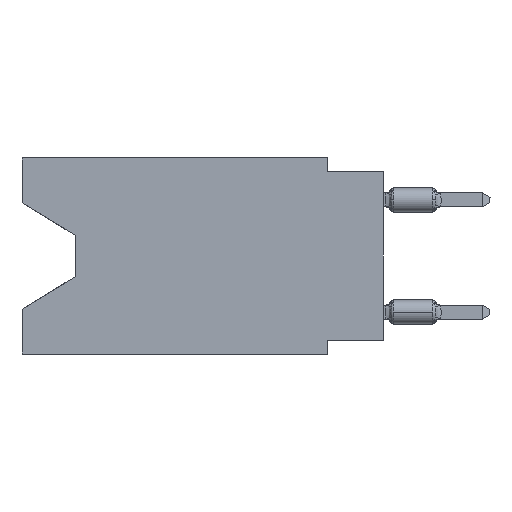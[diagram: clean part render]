
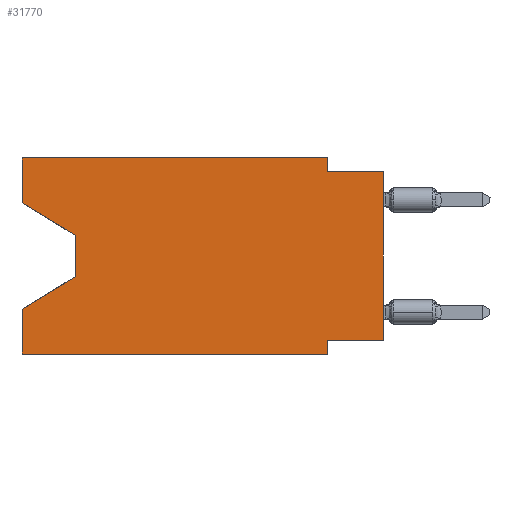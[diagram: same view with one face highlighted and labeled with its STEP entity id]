
A CAD part, left-side view. The second image highlights one B-rep face of the part: STEP entity #31770.
In plain terms, the highlighted planar face has unit normal (-1, 0, 0).
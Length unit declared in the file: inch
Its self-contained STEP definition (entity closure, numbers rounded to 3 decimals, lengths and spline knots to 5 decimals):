
#386 = DIRECTION ( 'NONE',  ( 1., 0., 0. ) ) ;
#463 = DIRECTION ( 'NONE',  ( 0., 0., 1. ) ) ;
#1813 = VECTOR ( 'NONE', #39213, 39.37008 ) ;
#2284 = VERTEX_POINT ( 'NONE', #43591 ) ;
#3440 = EDGE_CURVE ( 'NONE', #39043, #18679, #49309, .T. ) ;
#3689 = ORIENTED_EDGE ( 'NONE', *, *, #38426, .F. ) ;
#4699 = VECTOR ( 'NONE', #14234, 39.37008 ) ;
#5346 = CARTESIAN_POINT ( 'NONE',  ( 0., 0.645, -0.08025 ) ) ;
#5384 = CARTESIAN_POINT ( 'NONE',  ( 0., 0.1, -0.025 ) ) ;
#5559 = ORIENTED_EDGE ( 'NONE', *, *, #10562, .T. ) ;
#5564 = CARTESIAN_POINT ( 'NONE',  ( 0., 0.1, -0.35 ) ) ;
#5602 = DIRECTION ( 'NONE',  ( 0., -1., 0. ) ) ;
#5837 = LINE ( 'NONE', #22225, #13794 ) ;
#6562 = CARTESIAN_POINT ( 'NONE',  ( 0., 0.1, -0.35 ) ) ;
#6981 = CARTESIAN_POINT ( 'NONE',  ( 0., 0.645, -0.35 ) ) ;
#7416 = LINE ( 'NONE', #23812, #23748 ) ;
#8357 = EDGE_CURVE ( 'NONE', #27880, #24986, #37731, .T. ) ;
#8923 = DIRECTION ( 'NONE',  ( 0., 0., 1. ) ) ;
#9440 = LINE ( 'NONE', #12428, #40770 ) ;
#9547 = VECTOR ( 'NONE', #10209, 39.37008 ) ;
#9604 = LINE ( 'NONE', #26022, #52636 ) ;
#9800 = VERTEX_POINT ( 'NONE', #5564 ) ;
#10209 = DIRECTION ( 'NONE',  ( 0., 0., 1. ) ) ;
#10562 = EDGE_CURVE ( 'NONE', #45503, #2284, #9440, .T. ) ;
#10988 = VERTEX_POINT ( 'NONE', #50280 ) ;
#12251 = VECTOR ( 'NONE', #8923, 39.37008 ) ;
#12428 = CARTESIAN_POINT ( 'NONE',  ( 0., 0.55, -0.212 ) ) ;
#13794 = VECTOR ( 'NONE', #26280, 39.37008 ) ;
#13832 = ORIENTED_EDGE ( 'NONE', *, *, #48872, .F. ) ;
#14234 = DIRECTION ( 'NONE',  ( 0., -1., 0. ) ) ;
#15214 = LINE ( 'NONE', #22788, #1813 ) ;
#16140 = VERTEX_POINT ( 'NONE', #45741 ) ;
#16524 = DIRECTION ( 'NONE',  ( 0., 1., 0. ) ) ;
#18679 = VERTEX_POINT ( 'NONE', #5384 ) ;
#18775 = LINE ( 'NONE', #43043, #4699 ) ;
#19241 = VECTOR ( 'NONE', #21773, 39.37008 ) ;
#20510 = CARTESIAN_POINT ( 'NONE',  ( 0., 0.645, 0. ) ) ;
#21499 = CARTESIAN_POINT ( 'NONE',  ( 0., 0.55, -0.138 ) ) ;
#21773 = DIRECTION ( 'NONE',  ( 0., 0., -1. ) ) ;
#22225 = CARTESIAN_POINT ( 'NONE',  ( 0., 0.645, -0.35 ) ) ;
#22643 = ORIENTED_EDGE ( 'NONE', *, *, #25276, .T. ) ;
#22788 = CARTESIAN_POINT ( 'NONE',  ( 0., 0.645, -0.08025 ) ) ;
#23230 = ORIENTED_EDGE ( 'NONE', *, *, #36352, .F. ) ;
#23360 = ORIENTED_EDGE ( 'NONE', *, *, #43821, .T. ) ;
#23748 = VECTOR ( 'NONE', #16524, 39.37008 ) ;
#23812 = CARTESIAN_POINT ( 'NONE',  ( 0., 0., -0.325 ) ) ;
#24648 = ORIENTED_EDGE ( 'NONE', *, *, #8357, .T. ) ;
#24986 = VERTEX_POINT ( 'NONE', #38938 ) ;
#25276 = EDGE_CURVE ( 'NONE', #16140, #45503, #30129, .T. ) ;
#26022 = CARTESIAN_POINT ( 'NONE',  ( 0., 0.645, 0. ) ) ;
#26280 = DIRECTION ( 'NONE',  ( 0., -1., 0. ) ) ;
#26808 = CARTESIAN_POINT ( 'NONE',  ( 0., 0.1, 0. ) ) ;
#26828 = ORIENTED_EDGE ( 'NONE', *, *, #41934, .T. ) ;
#27648 = VECTOR ( 'NONE', #43235, 39.37008 ) ;
#27691 = VERTEX_POINT ( 'NONE', #6981 ) ;
#27880 = VERTEX_POINT ( 'NONE', #36312 ) ;
#28951 = LINE ( 'NONE', #49660, #36181 ) ;
#30027 = ORIENTED_EDGE ( 'NONE', *, *, #42074, .F. ) ;
#30129 = LINE ( 'NONE', #21499, #19241 ) ;
#31222 = ORIENTED_EDGE ( 'NONE', *, *, #41468, .F. ) ;
#31770 = ADVANCED_FACE ( 'NONE', ( #40521 ), #52617, .F. ) ;
#32795 = VERTEX_POINT ( 'NONE', #5346 ) ;
#33426 = CARTESIAN_POINT ( 'NONE',  ( 0., 0., 0. ) ) ;
#33681 = DIRECTION ( 'NONE',  ( 0., 0.855, -0.519 ) ) ;
#36181 = VECTOR ( 'NONE', #463, 39.37008 ) ;
#36312 = CARTESIAN_POINT ( 'NONE',  ( 0., 0., -0.325 ) ) ;
#36352 = EDGE_CURVE ( 'NONE', #40684, #39043, #9604, .T. ) ;
#37537 = EDGE_CURVE ( 'NONE', #10988, #9800, #47181, .T. ) ;
#37731 = LINE ( 'NONE', #33426, #12251 ) ;
#38330 = ORIENTED_EDGE ( 'NONE', *, *, #37537, .F. ) ;
#38426 = EDGE_CURVE ( 'NONE', #18679, #24986, #18775, .T. ) ;
#38938 = CARTESIAN_POINT ( 'NONE',  ( 0., 0., -0.025 ) ) ;
#39043 = VERTEX_POINT ( 'NONE', #42073 ) ;
#39213 = DIRECTION ( 'NONE',  ( 0., -0.855, -0.519 ) ) ;
#39640 = DIRECTION ( 'NONE',  ( 0., 0., -1. ) ) ;
#40233 = CARTESIAN_POINT ( 'NONE',  ( 0., 0.55, -0.212 ) ) ;
#40521 = FACE_OUTER_BOUND ( 'NONE', #51322, .T. ) ;
#40684 = VERTEX_POINT ( 'NONE', #20510 ) ;
#40770 = VECTOR ( 'NONE', #33681, 39.37008 ) ;
#41468 = EDGE_CURVE ( 'NONE', #32795, #40684, #43316, .T. ) ;
#41818 = CARTESIAN_POINT ( 'NONE',  ( 0., 0.645, 0. ) ) ;
#41934 = EDGE_CURVE ( 'NONE', #32795, #16140, #15214, .T. ) ;
#42073 = CARTESIAN_POINT ( 'NONE',  ( 0., 0.1, 0. ) ) ;
#42074 = EDGE_CURVE ( 'NONE', #27691, #2284, #28951, .T. ) ;
#43043 = CARTESIAN_POINT ( 'NONE',  ( 0., 0., -0.025 ) ) ;
#43235 = DIRECTION ( 'NONE',  ( 0., 0., -1. ) ) ;
#43316 = LINE ( 'NONE', #44104, #9547 ) ;
#43591 = CARTESIAN_POINT ( 'NONE',  ( 0., 0.645, -0.26975 ) ) ;
#43821 = EDGE_CURVE ( 'NONE', #27691, #9800, #5837, .T. ) ;
#44104 = CARTESIAN_POINT ( 'NONE',  ( 0., 0.645, 0. ) ) ;
#45503 = VERTEX_POINT ( 'NONE', #40233 ) ;
#45741 = CARTESIAN_POINT ( 'NONE',  ( 0., 0.55, -0.138 ) ) ;
#46884 = AXIS2_PLACEMENT_3D ( 'NONE', #41818, #386, #50105 ) ;
#47181 = LINE ( 'NONE', #6562, #48408 ) ;
#48408 = VECTOR ( 'NONE', #39640, 39.37008 ) ;
#48872 = EDGE_CURVE ( 'NONE', #27880, #10988, #7416, .T. ) ;
#49309 = LINE ( 'NONE', #26808, #27648 ) ;
#49660 = CARTESIAN_POINT ( 'NONE',  ( 0., 0.645, 0. ) ) ;
#50105 = DIRECTION ( 'NONE',  ( 0., 0., -1. ) ) ;
#50280 = CARTESIAN_POINT ( 'NONE',  ( 0., 0.1, -0.325 ) ) ;
#51322 = EDGE_LOOP ( 'NONE', ( #26828, #22643, #5559, #30027, #23360, #38330, #13832, #24648, #3689, #51574, #23230, #31222 ) ) ;
#51574 = ORIENTED_EDGE ( 'NONE', *, *, #3440, .F. ) ;
#52617 = PLANE ( 'NONE',  #46884 ) ;
#52636 = VECTOR ( 'NONE', #5602, 39.37008 ) ;
